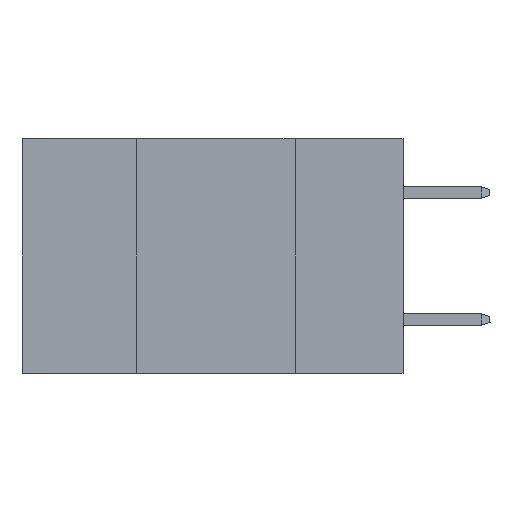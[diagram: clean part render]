
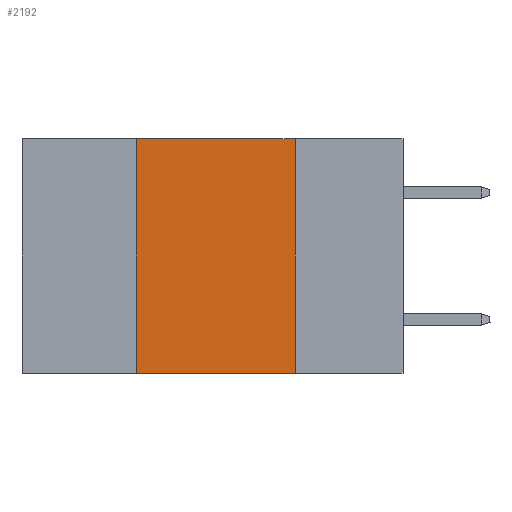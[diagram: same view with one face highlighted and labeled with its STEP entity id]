
A CAD part, left-side view. The second image highlights one B-rep face of the part: STEP entity #2192.
In plain terms, the highlighted planar face has unit normal (-1, 0, 0).
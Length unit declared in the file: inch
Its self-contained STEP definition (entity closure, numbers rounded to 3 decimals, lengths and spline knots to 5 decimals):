
#470 = VECTOR ( 'NONE', #9332, 39.37008 ) ;
#1052 = ORIENTED_EDGE ( 'NONE', *, *, #4030, .F. ) ;
#1712 = LINE ( 'NONE', #9590, #10011 ) ;
#2192 = ADVANCED_FACE ( 'NONE', ( #5400 ), #19083, .F. ) ;
#4030 = EDGE_CURVE ( 'NONE', #12399, #4392, #1712, .T. ) ;
#4276 = CARTESIAN_POINT ( 'NONE',  ( 0., 0.42, 0. ) ) ;
#4392 = VERTEX_POINT ( 'NONE', #21676 ) ;
#5400 = FACE_OUTER_BOUND ( 'NONE', #19327, .T. ) ;
#5530 = CARTESIAN_POINT ( 'NONE',  ( 0., 0.6, 0. ) ) ;
#7261 = CARTESIAN_POINT ( 'NONE',  ( 0., 0.6, 0. ) ) ;
#7563 = CARTESIAN_POINT ( 'NONE',  ( 0., 0.42, -0.37 ) ) ;
#8725 = VERTEX_POINT ( 'NONE', #7563 ) ;
#9332 = DIRECTION ( 'NONE',  ( 0., -1., 0. ) ) ;
#9399 = EDGE_CURVE ( 'NONE', #8725, #4392, #17080, .T. ) ;
#9590 = CARTESIAN_POINT ( 'NONE',  ( 0., 0.17, 0. ) ) ;
#9810 = LINE ( 'NONE', #4276, #12377 ) ;
#10011 = VECTOR ( 'NONE', #21327, 39.37008 ) ;
#10533 = EDGE_CURVE ( 'NONE', #8725, #13742, #9810, .T. ) ;
#10908 = ORIENTED_EDGE ( 'NONE', *, *, #10533, .F. ) ;
#11146 = LINE ( 'NONE', #7261, #470 ) ;
#11228 = CARTESIAN_POINT ( 'NONE',  ( 0., 0.6, -0.37 ) ) ;
#12120 = DIRECTION ( 'NONE',  ( 0., 0., 1. ) ) ;
#12377 = VECTOR ( 'NONE', #12120, 39.37008 ) ;
#12399 = VERTEX_POINT ( 'NONE', #18910 ) ;
#12606 = AXIS2_PLACEMENT_3D ( 'NONE', #5530, #24994, #15259 ) ;
#13742 = VERTEX_POINT ( 'NONE', #15312 ) ;
#14684 = DIRECTION ( 'NONE',  ( 0., -1., 0. ) ) ;
#15259 = DIRECTION ( 'NONE',  ( 0., 0., -1. ) ) ;
#15312 = CARTESIAN_POINT ( 'NONE',  ( 0., 0.42, 0. ) ) ;
#17080 = LINE ( 'NONE', #11228, #18448 ) ;
#17426 = ORIENTED_EDGE ( 'NONE', *, *, #9399, .T. ) ;
#18448 = VECTOR ( 'NONE', #14684, 39.37008 ) ;
#18910 = CARTESIAN_POINT ( 'NONE',  ( 0., 0.17, 0. ) ) ;
#19083 = PLANE ( 'NONE',  #12606 ) ;
#19327 = EDGE_LOOP ( 'NONE', ( #1052, #20111, #10908, #17426 ) ) ;
#20111 = ORIENTED_EDGE ( 'NONE', *, *, #22705, .F. ) ;
#21327 = DIRECTION ( 'NONE',  ( 0., 0., -1. ) ) ;
#21676 = CARTESIAN_POINT ( 'NONE',  ( 0., 0.17, -0.37 ) ) ;
#22705 = EDGE_CURVE ( 'NONE', #13742, #12399, #11146, .T. ) ;
#24994 = DIRECTION ( 'NONE',  ( 1., 0., 0. ) ) ;
